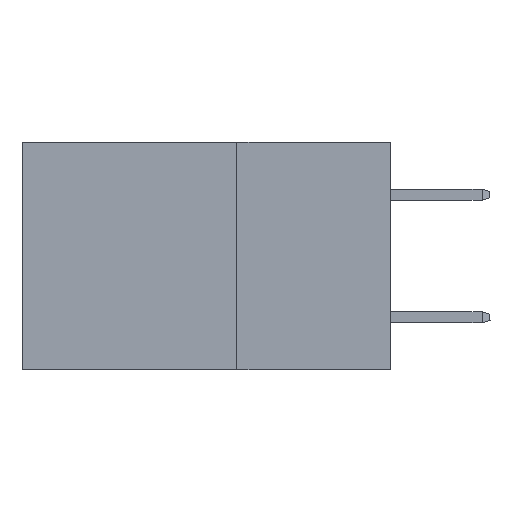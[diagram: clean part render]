
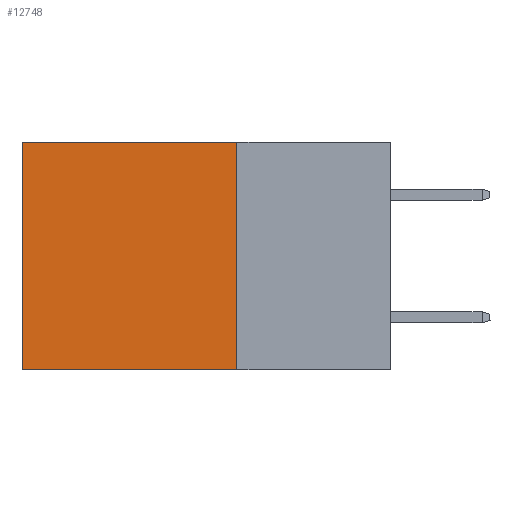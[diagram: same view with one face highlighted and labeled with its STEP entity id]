
A CAD part, left-side view. The second image highlights one B-rep face of the part: STEP entity #12748.
In plain terms, the highlighted planar face has unit normal (-1, 0, 0).
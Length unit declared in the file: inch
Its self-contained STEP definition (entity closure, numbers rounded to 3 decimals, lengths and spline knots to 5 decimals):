
#2340 = EDGE_CURVE ( 'NONE', #3900, #4830, #17275, .T. ) ;
#2669 = EDGE_LOOP ( 'NONE', ( #11836, #26232, #20452, #16668 ) ) ;
#3306 = DIRECTION ( 'NONE',  ( 0., 0., -1. ) ) ;
#3355 = PLANE ( 'NONE',  #19827 ) ;
#3792 = DIRECTION ( 'NONE',  ( 0., 1., 0. ) ) ;
#3900 = VERTEX_POINT ( 'NONE', #20512 ) ;
#4830 = VERTEX_POINT ( 'NONE', #6526 ) ;
#4867 = VECTOR ( 'NONE', #3792, 39.37008 ) ;
#5196 = EDGE_CURVE ( 'NONE', #9991, #17185, #9500, .T. ) ;
#5592 = DIRECTION ( 'NONE',  ( 0., 0., -1. ) ) ;
#6526 = CARTESIAN_POINT ( 'NONE',  ( 0.2875, 0.6, -0.37 ) ) ;
#7609 = CARTESIAN_POINT ( 'NONE',  ( 0.2875, 0.25, 0. ) ) ;
#8051 = EDGE_CURVE ( 'NONE', #17185, #4830, #15372, .T. ) ;
#9500 = LINE ( 'NONE', #10377, #20533 ) ;
#9760 = FACE_OUTER_BOUND ( 'NONE', #2669, .T. ) ;
#9991 = VERTEX_POINT ( 'NONE', #14032 ) ;
#10377 = CARTESIAN_POINT ( 'NONE',  ( 0.2875, 0.25, 0. ) ) ;
#11836 = ORIENTED_EDGE ( 'NONE', *, *, #8051, .T. ) ;
#12748 = ADVANCED_FACE ( 'NONE', ( #9760 ), #3355, .F. ) ;
#14032 = CARTESIAN_POINT ( 'NONE',  ( 0.2875, 0.25, 0. ) ) ;
#14338 = VECTOR ( 'NONE', #24815, 39.37008 ) ;
#14618 = DIRECTION ( 'NONE',  ( 0., 1., 0. ) ) ;
#15372 = LINE ( 'NONE', #20129, #14338 ) ;
#16454 = DIRECTION ( 'NONE',  ( 1., 0., 0. ) ) ;
#16496 = CARTESIAN_POINT ( 'NONE',  ( 0.2875, 0.25, 0. ) ) ;
#16668 = ORIENTED_EDGE ( 'NONE', *, *, #5196, .T. ) ;
#17185 = VERTEX_POINT ( 'NONE', #21846 ) ;
#17275 = LINE ( 'NONE', #22925, #4867 ) ;
#18723 = LINE ( 'NONE', #16496, #24183 ) ;
#19827 = AXIS2_PLACEMENT_3D ( 'NONE', #7609, #16454, #5592 ) ;
#20129 = CARTESIAN_POINT ( 'NONE',  ( 0.2875, 0.6, 0. ) ) ;
#20452 = ORIENTED_EDGE ( 'NONE', *, *, #20841, .F. ) ;
#20512 = CARTESIAN_POINT ( 'NONE',  ( 0.2875, 0.25, -0.37 ) ) ;
#20533 = VECTOR ( 'NONE', #14618, 39.37008 ) ;
#20841 = EDGE_CURVE ( 'NONE', #9991, #3900, #18723, .T. ) ;
#21846 = CARTESIAN_POINT ( 'NONE',  ( 0.2875, 0.6, 0. ) ) ;
#22925 = CARTESIAN_POINT ( 'NONE',  ( 0.2875, 0.25, -0.37 ) ) ;
#24183 = VECTOR ( 'NONE', #3306, 39.37008 ) ;
#24815 = DIRECTION ( 'NONE',  ( 0., 0., -1. ) ) ;
#26232 = ORIENTED_EDGE ( 'NONE', *, *, #2340, .F. ) ;
